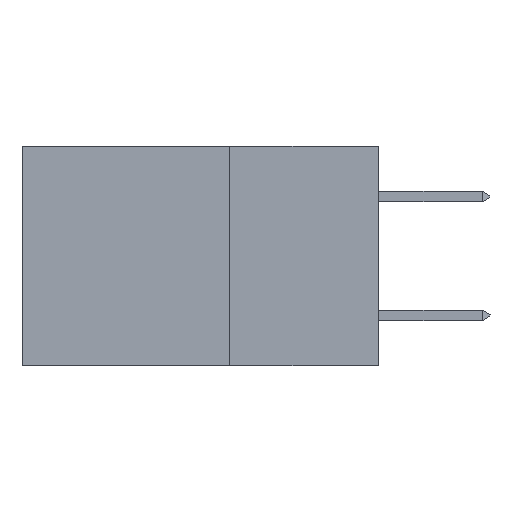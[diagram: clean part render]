
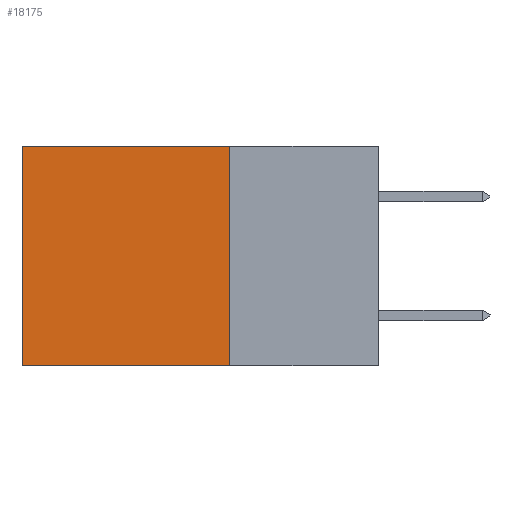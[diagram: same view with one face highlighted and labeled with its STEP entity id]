
A CAD part, left-side view. The second image highlights one B-rep face of the part: STEP entity #18175.
In plain terms, the highlighted planar face has unit normal (-1, 0, 0).
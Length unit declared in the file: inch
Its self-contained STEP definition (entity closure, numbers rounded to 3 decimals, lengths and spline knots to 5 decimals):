
#602 = ORIENTED_EDGE ( 'NONE', *, *, #16767, .F. ) ;
#1110 = VECTOR ( 'NONE', #15817, 39.37008 ) ;
#1212 = CARTESIAN_POINT ( 'NONE',  ( 0.298, 0.25, -0.37 ) ) ;
#1432 = CARTESIAN_POINT ( 'NONE',  ( 0.298, 0.25, 0. ) ) ;
#2316 = CARTESIAN_POINT ( 'NONE',  ( 0.298, 0.25, 0. ) ) ;
#3499 = CARTESIAN_POINT ( 'NONE',  ( 0.298, 0.6, -0.37 ) ) ;
#3637 = ORIENTED_EDGE ( 'NONE', *, *, #16020, .F. ) ;
#4516 = FACE_OUTER_BOUND ( 'NONE', #12423, .T. ) ;
#5267 = AXIS2_PLACEMENT_3D ( 'NONE', #2316, #8161, #21242 ) ;
#6080 = VECTOR ( 'NONE', #8848, 39.37008 ) ;
#7187 = CARTESIAN_POINT ( 'NONE',  ( 0.298, 0.25, 0. ) ) ;
#7440 = DIRECTION ( 'NONE',  ( 0., 1., 0. ) ) ;
#8161 = DIRECTION ( 'NONE',  ( 1., 0., 0. ) ) ;
#8379 = LINE ( 'NONE', #10074, #1110 ) ;
#8848 = DIRECTION ( 'NONE',  ( 0., 1., 0. ) ) ;
#10074 = CARTESIAN_POINT ( 'NONE',  ( 0.298, 0.25, 0. ) ) ;
#11353 = VERTEX_POINT ( 'NONE', #3499 ) ;
#11954 = LINE ( 'NONE', #12704, #6080 ) ;
#12423 = EDGE_LOOP ( 'NONE', ( #21487, #3637, #602, #16382 ) ) ;
#12682 = CARTESIAN_POINT ( 'NONE',  ( 0.298, 0.6, 0. ) ) ;
#12704 = CARTESIAN_POINT ( 'NONE',  ( 0.298, 0.25, -0.37 ) ) ;
#13580 = PLANE ( 'NONE',  #5267 ) ;
#14035 = CARTESIAN_POINT ( 'NONE',  ( 0.298, 0.6, 0. ) ) ;
#15817 = DIRECTION ( 'NONE',  ( 0., 0., -1. ) ) ;
#16020 = EDGE_CURVE ( 'NONE', #17160, #11353, #11954, .T. ) ;
#16181 = DIRECTION ( 'NONE',  ( 0., 0., -1. ) ) ;
#16382 = ORIENTED_EDGE ( 'NONE', *, *, #20905, .T. ) ;
#16767 = EDGE_CURVE ( 'NONE', #16888, #17160, #8379, .T. ) ;
#16888 = VERTEX_POINT ( 'NONE', #1432 ) ;
#17160 = VERTEX_POINT ( 'NONE', #1212 ) ;
#17756 = VECTOR ( 'NONE', #16181, 39.37008 ) ;
#18175 = ADVANCED_FACE ( 'NONE', ( #4516 ), #13580, .F. ) ;
#18626 = VECTOR ( 'NONE', #7440, 39.37008 ) ;
#20645 = LINE ( 'NONE', #7187, #18626 ) ;
#20837 = EDGE_CURVE ( 'NONE', #21664, #11353, #23600, .T. ) ;
#20905 = EDGE_CURVE ( 'NONE', #16888, #21664, #20645, .T. ) ;
#21242 = DIRECTION ( 'NONE',  ( 0., 0., -1. ) ) ;
#21487 = ORIENTED_EDGE ( 'NONE', *, *, #20837, .T. ) ;
#21664 = VERTEX_POINT ( 'NONE', #14035 ) ;
#23600 = LINE ( 'NONE', #12682, #17756 ) ;
